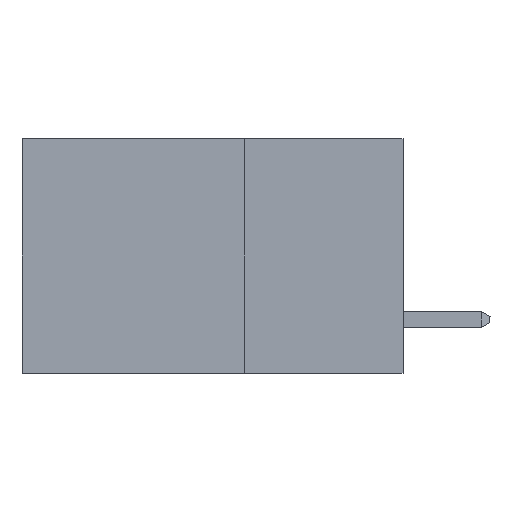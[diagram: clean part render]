
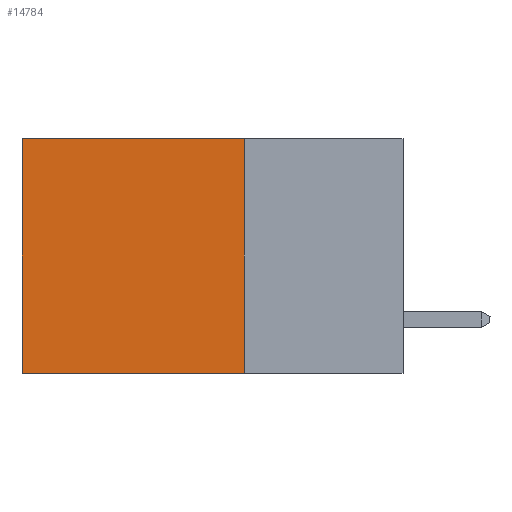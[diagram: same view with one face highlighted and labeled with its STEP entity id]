
A CAD part, left-side view. The second image highlights one B-rep face of the part: STEP entity #14784.
In plain terms, the highlighted planar face has unit normal (-1, 0, 0).
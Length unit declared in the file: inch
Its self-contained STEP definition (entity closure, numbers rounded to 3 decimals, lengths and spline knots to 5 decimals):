
#2012 = LINE ( 'NONE', #11471, #22025 ) ;
#2521 = DIRECTION ( 'NONE',  ( 0., 0., -1. ) ) ;
#2680 = VERTEX_POINT ( 'NONE', #6148 ) ;
#3093 = EDGE_CURVE ( 'NONE', #5775, #18238, #19561, .T. ) ;
#3695 = ORIENTED_EDGE ( 'NONE', *, *, #21138, .F. ) ;
#4078 = CARTESIAN_POINT ( 'NONE',  ( 0.2875, 0.25, -0.37 ) ) ;
#4901 = ORIENTED_EDGE ( 'NONE', *, *, #21297, .F. ) ;
#5198 = DIRECTION ( 'NONE',  ( 0., 0., -1. ) ) ;
#5775 = VERTEX_POINT ( 'NONE', #7252 ) ;
#6148 = CARTESIAN_POINT ( 'NONE',  ( 0.2875, 0.6, -0.37 ) ) ;
#6250 = VECTOR ( 'NONE', #17840, 39.37008 ) ;
#7252 = CARTESIAN_POINT ( 'NONE',  ( 0.2875, 0.25, 0. ) ) ;
#8903 = EDGE_LOOP ( 'NONE', ( #19837, #3695, #4901, #18444 ) ) ;
#9243 = PLANE ( 'NONE',  #13641 ) ;
#9552 = LINE ( 'NONE', #24061, #25555 ) ;
#11230 = DIRECTION ( 'NONE',  ( 0., 0., -1. ) ) ;
#11471 = CARTESIAN_POINT ( 'NONE',  ( 0.2875, 0.25, -0.37 ) ) ;
#12066 = CARTESIAN_POINT ( 'NONE',  ( 0.2875, 0.25, 0. ) ) ;
#13641 = AXIS2_PLACEMENT_3D ( 'NONE', #16285, #20708, #11230 ) ;
#13680 = FACE_OUTER_BOUND ( 'NONE', #8903, .T. ) ;
#14784 = ADVANCED_FACE ( 'NONE', ( #13680 ), #9243, .F. ) ;
#16285 = CARTESIAN_POINT ( 'NONE',  ( 0.2875, 0.25, 0. ) ) ;
#16514 = DIRECTION ( 'NONE',  ( 0., 1., 0. ) ) ;
#17840 = DIRECTION ( 'NONE',  ( 0., 1., 0. ) ) ;
#18238 = VERTEX_POINT ( 'NONE', #23129 ) ;
#18444 = ORIENTED_EDGE ( 'NONE', *, *, #3093, .T. ) ;
#19561 = LINE ( 'NONE', #24010, #6250 ) ;
#19704 = LINE ( 'NONE', #12066, #27413 ) ;
#19837 = ORIENTED_EDGE ( 'NONE', *, *, #29518, .T. ) ;
#20708 = DIRECTION ( 'NONE',  ( 1., 0., 0. ) ) ;
#21138 = EDGE_CURVE ( 'NONE', #23098, #2680, #2012, .T. ) ;
#21297 = EDGE_CURVE ( 'NONE', #5775, #23098, #19704, .T. ) ;
#22025 = VECTOR ( 'NONE', #16514, 39.37008 ) ;
#23098 = VERTEX_POINT ( 'NONE', #4078 ) ;
#23129 = CARTESIAN_POINT ( 'NONE',  ( 0.2875, 0.6, 0. ) ) ;
#24010 = CARTESIAN_POINT ( 'NONE',  ( 0.2875, 0.25, 0. ) ) ;
#24061 = CARTESIAN_POINT ( 'NONE',  ( 0.2875, 0.6, 0. ) ) ;
#25555 = VECTOR ( 'NONE', #2521, 39.37008 ) ;
#27413 = VECTOR ( 'NONE', #5198, 39.37008 ) ;
#29518 = EDGE_CURVE ( 'NONE', #18238, #2680, #9552, .T. ) ;
